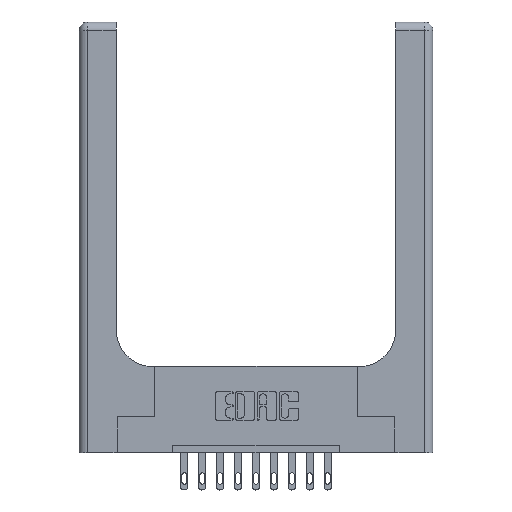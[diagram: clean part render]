
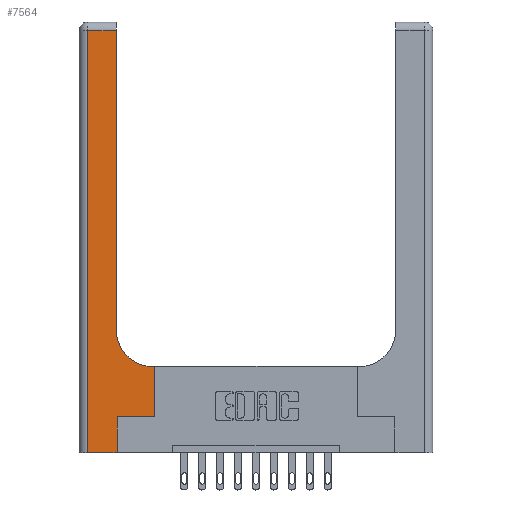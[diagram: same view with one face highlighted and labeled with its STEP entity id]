
A CAD part, top view. The second image highlights one B-rep face of the part: STEP entity #7564.
In plain terms, the highlighted planar face has unit normal (0, 0, 1).
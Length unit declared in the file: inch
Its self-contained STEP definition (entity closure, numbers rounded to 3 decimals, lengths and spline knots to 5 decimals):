
#348 = AXIS2_PLACEMENT_3D ( 'NONE', #9120, #699, #4145 ) ;
#699 = DIRECTION ( 'NONE',  ( 0., 0., -1. ) ) ;
#710 = CARTESIAN_POINT ( 'NONE',  ( 0., 0., 0.37 ) ) ;
#896 = EDGE_CURVE ( 'NONE', #13857, #12301, #14534, .T. ) ;
#1158 = CARTESIAN_POINT ( 'NONE',  ( 0.265, 0.25, 0.37 ) ) ;
#1378 = VECTOR ( 'NONE', #10386, 39.37008 ) ;
#1501 = VECTOR ( 'NONE', #7978, 39.37008 ) ;
#1533 = LINE ( 'NONE', #4994, #2251 ) ;
#1574 = CARTESIAN_POINT ( 'NONE',  ( 0., 2.94, 0.37 ) ) ;
#1640 = ORIENTED_EDGE ( 'NONE', *, *, #2471, .T. ) ;
#1951 = CARTESIAN_POINT ( 'NONE',  ( 0.26, 0.85, 0.37 ) ) ;
#1984 = VERTEX_POINT ( 'NONE', #6773 ) ;
#2036 = VECTOR ( 'NONE', #9057, 39.37008 ) ;
#2038 = LINE ( 'NONE', #710, #1378 ) ;
#2106 = FACE_OUTER_BOUND ( 'NONE', #12859, .T. ) ;
#2209 = ORIENTED_EDGE ( 'NONE', *, *, #13948, .T. ) ;
#2251 = VECTOR ( 'NONE', #6490, 39.37008 ) ;
#2356 = CIRCLE ( 'NONE', #4862, 0.25 ) ;
#2471 = EDGE_CURVE ( 'NONE', #13176, #13857, #12984, .T. ) ;
#2588 = DIRECTION ( 'NONE',  ( 0., 0., -1. ) ) ;
#2700 = VERTEX_POINT ( 'NONE', #4768 ) ;
#3362 = CARTESIAN_POINT ( 'NONE',  ( 0.528, 0.25, 0.37 ) ) ;
#3399 = VERTEX_POINT ( 'NONE', #10557 ) ;
#4145 = DIRECTION ( 'NONE',  ( -1., 0., 0. ) ) ;
#4768 = CARTESIAN_POINT ( 'NONE',  ( 0.26, 2.94, 0.37 ) ) ;
#4811 = ORIENTED_EDGE ( 'NONE', *, *, #10049, .T. ) ;
#4837 = DIRECTION ( 'NONE',  ( 1., 0., 0. ) ) ;
#4862 = AXIS2_PLACEMENT_3D ( 'NONE', #9841, #2588, #14777 ) ;
#4994 = CARTESIAN_POINT ( 'NONE',  ( 0.26, 3., 0.37 ) ) ;
#5547 = ORIENTED_EDGE ( 'NONE', *, *, #13288, .T. ) ;
#5615 = EDGE_CURVE ( 'NONE', #1984, #11106, #8050, .T. ) ;
#5750 = VECTOR ( 'NONE', #4837, 39.37008 ) ;
#6490 = DIRECTION ( 'NONE',  ( 0., 1., 0. ) ) ;
#6691 = LINE ( 'NONE', #1574, #2036 ) ;
#6773 = CARTESIAN_POINT ( 'NONE',  ( 0.06, 2.94, 0.37 ) ) ;
#7166 = ORIENTED_EDGE ( 'NONE', *, *, #12063, .T. ) ;
#7564 = ADVANCED_FACE ( 'NONE', ( #2106 ), #9200, .F. ) ;
#7578 = DIRECTION ( 'NONE',  ( -1., 0., 0. ) ) ;
#7937 = VECTOR ( 'NONE', #7578, 39.37008 ) ;
#7978 = DIRECTION ( 'NONE',  ( 0., -1., 0. ) ) ;
#8050 = LINE ( 'NONE', #13965, #1501 ) ;
#8151 = EDGE_CURVE ( 'NONE', #15018, #2700, #1533, .T. ) ;
#8328 = CARTESIAN_POINT ( 'NONE',  ( 0.265, 0., 0.37 ) ) ;
#8432 = ORIENTED_EDGE ( 'NONE', *, *, #8151, .T. ) ;
#8493 = EDGE_CURVE ( 'NONE', #2700, #1984, #6691, .T. ) ;
#8494 = CARTESIAN_POINT ( 'NONE',  ( 0.528, 0.25, 0.37 ) ) ;
#9057 = DIRECTION ( 'NONE',  ( -1., 0., 0. ) ) ;
#9120 = CARTESIAN_POINT ( 'NONE',  ( 0., 3., 0.37 ) ) ;
#9200 = PLANE ( 'NONE',  #348 ) ;
#9665 = VECTOR ( 'NONE', #14230, 39.37008 ) ;
#9841 = CARTESIAN_POINT ( 'NONE',  ( 0.51, 0.85, 0.37 ) ) ;
#9886 = LINE ( 'NONE', #13285, #7937 ) ;
#10049 = EDGE_CURVE ( 'NONE', #12301, #3399, #12108, .T. ) ;
#10266 = ORIENTED_EDGE ( 'NONE', *, *, #5615, .T. ) ;
#10386 = DIRECTION ( 'NONE',  ( 1., 0., 0. ) ) ;
#10528 = CARTESIAN_POINT ( 'NONE',  ( 0.265, 0.25, 0.37 ) ) ;
#10557 = CARTESIAN_POINT ( 'NONE',  ( 0.528, 0.6, 0.37 ) ) ;
#11106 = VERTEX_POINT ( 'NONE', #11434 ) ;
#11314 = ORIENTED_EDGE ( 'NONE', *, *, #896, .T. ) ;
#11378 = VECTOR ( 'NONE', #14541, 39.37008 ) ;
#11434 = CARTESIAN_POINT ( 'NONE',  ( 0.06, 0., 0.37 ) ) ;
#12063 = EDGE_CURVE ( 'NONE', #12359, #15018, #2356, .T. ) ;
#12108 = LINE ( 'NONE', #8494, #11378 ) ;
#12301 = VERTEX_POINT ( 'NONE', #3362 ) ;
#12359 = VERTEX_POINT ( 'NONE', #13299 ) ;
#12859 = EDGE_LOOP ( 'NONE', ( #8432, #13624, #10266, #5547, #1640, #11314, #4811, #2209, #7166 ) ) ;
#12984 = LINE ( 'NONE', #8328, #9665 ) ;
#13176 = VERTEX_POINT ( 'NONE', #13548 ) ;
#13285 = CARTESIAN_POINT ( 'NONE',  ( 0.26, 0.6, 0.37 ) ) ;
#13288 = EDGE_CURVE ( 'NONE', #11106, #13176, #2038, .T. ) ;
#13299 = CARTESIAN_POINT ( 'NONE',  ( 0.51, 0.6, 0.37 ) ) ;
#13548 = CARTESIAN_POINT ( 'NONE',  ( 0.265, 0., 0.37 ) ) ;
#13624 = ORIENTED_EDGE ( 'NONE', *, *, #8493, .T. ) ;
#13857 = VERTEX_POINT ( 'NONE', #10528 ) ;
#13948 = EDGE_CURVE ( 'NONE', #3399, #12359, #9886, .T. ) ;
#13965 = CARTESIAN_POINT ( 'NONE',  ( 0.06, 3., 0.37 ) ) ;
#14230 = DIRECTION ( 'NONE',  ( 0., 1., 0. ) ) ;
#14534 = LINE ( 'NONE', #1158, #5750 ) ;
#14541 = DIRECTION ( 'NONE',  ( 0., 1., 0. ) ) ;
#14777 = DIRECTION ( 'NONE',  ( 1., 0., 0. ) ) ;
#15018 = VERTEX_POINT ( 'NONE', #1951 ) ;
